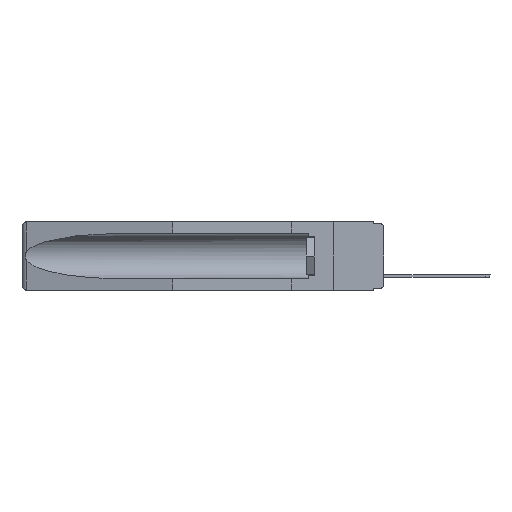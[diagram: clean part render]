
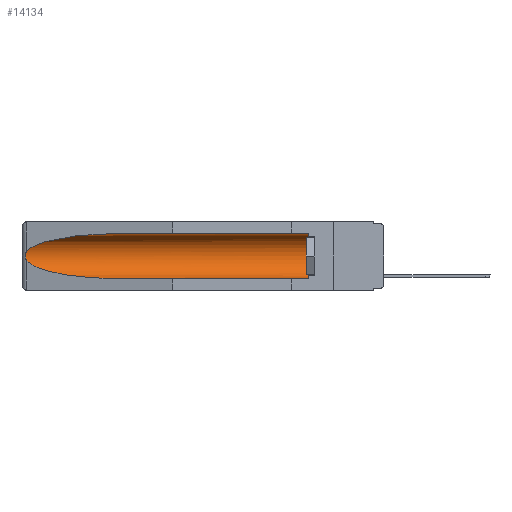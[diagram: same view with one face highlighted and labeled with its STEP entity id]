
A CAD part, left-side view. The second image highlights one B-rep face of the part: STEP entity #14134.
In plain terms, the highlighted cylindrical face has radius 2.857 mm (diameter 5.715 mm), a partial arc.
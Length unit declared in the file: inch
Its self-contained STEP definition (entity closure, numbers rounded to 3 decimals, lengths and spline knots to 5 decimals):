
#283 = EDGE_CURVE ( 'NONE', #15551, #11050, #1212, .T. ) ;
#292 = CARTESIAN_POINT ( 'NONE',  ( 0.26597, 1.5296, -0.19026 ) ) ;
#333 = CARTESIAN_POINT ( 'NONE',  ( 0.155, 1.07973, -0.284 ) ) ;
#392 = CARTESIAN_POINT ( 'NONE',  ( 0.155, 0.126, -0.1715 ) ) ;
#1212 =( BOUNDED_CURVE ( )  B_SPLINE_CURVE ( 3, ( #18219, #14955, #18429, #333 ),
 .UNSPECIFIED., .F., .F. ) 
 B_SPLINE_CURVE_WITH_KNOTS ( ( 4, 4 ),
 ( 0.1948, 1.5708 ),
 .UNSPECIFIED. ) 
 CURVE ( )  GEOMETRIC_REPRESENTATION_ITEM ( )  RATIONAL_B_SPLINE_CURVE ( ( 1., 0.848, 0.848, 1. ) ) 
 REPRESENTATION_ITEM ( '' )  );
#1786 = DIRECTION ( 'NONE',  ( 0., 0., 1. ) ) ;
#2035 = DIRECTION ( 'NONE',  ( 0., 0., 1. ) ) ;
#4675 = DIRECTION ( 'NONE',  ( 0., 1., 0. ) ) ;
#5060 = FACE_OUTER_BOUND ( 'NONE', #14733, .T. ) ;
#5086 = CARTESIAN_POINT ( 'NONE',  ( 0.26537, 1.52718, -0.19328 ) ) ;
#5282 = CARTESIAN_POINT ( 'NONE',  ( 0.26654, 1.53092, -0.15636 ) ) ;
#5899 = EDGE_CURVE ( 'NONE', #21203, #11050, #11670, .T. ) ;
#6003 = CARTESIAN_POINT ( 'NONE',  ( 0.26537, 1.52718, -0.14972 ) ) ;
#6364 = CARTESIAN_POINT ( 'NONE',  ( 0.26537, 1.52718, -0.19328 ) ) ;
#7251 = AXIS2_PLACEMENT_3D ( 'NONE', #392, #8354, #2035 ) ;
#7494 = VERTEX_POINT ( 'NONE', #12966 ) ;
#7540 = CARTESIAN_POINT ( 'NONE',  ( 0.21114, 1.30732, -0.059 ) ) ;
#7868 = ORIENTED_EDGE ( 'NONE', *, *, #19672, .T. ) ;
#7969 = ORIENTED_EDGE ( 'NONE', *, *, #15896, .T. ) ;
#8354 = DIRECTION ( 'NONE',  ( 0., -1., 0. ) ) ;
#8452 = CARTESIAN_POINT ( 'NONE',  ( 0.26597, 1.52961, -0.15275 ) ) ;
#8884 = CARTESIAN_POINT ( 'NONE',  ( 0.2673, 1.5327, -0.16383 ) ) ;
#8929 = ORIENTED_EDGE ( 'NONE', *, *, #16519, .T. ) ;
#9160 = CARTESIAN_POINT ( 'NONE',  ( 0.155, 1.07973, -0.059 ) ) ;
#10077 = ORIENTED_EDGE ( 'NONE', *, *, #12152, .T. ) ;
#10085 = CARTESIAN_POINT ( 'NONE',  ( 0.26655, 1.53094, -0.18657 ) ) ;
#11050 = VERTEX_POINT ( 'NONE', #17052 ) ;
#11521 = LINE ( 'NONE', #21470, #18979 ) ;
#11670 = LINE ( 'NONE', #13609, #13243 ) ;
#11712 = CARTESIAN_POINT ( 'NONE',  ( 0.155, -0.30754, -0.1715 ) ) ;
#12152 = EDGE_CURVE ( 'NONE', #16739, #17936, #11521, .T. ) ;
#12517 = ORIENTED_EDGE ( 'NONE', *, *, #5899, .F. ) ;
#12966 = CARTESIAN_POINT ( 'NONE',  ( 0.26537, 1.52718, -0.14972 ) ) ;
#13243 = VECTOR ( 'NONE', #18323, 39.37008 ) ;
#13474 = CARTESIAN_POINT ( 'NONE',  ( 0.26537, 1.52718, -0.14972 ) ) ;
#13591 = CARTESIAN_POINT ( 'NONE',  ( 0.155, 1.07973, -0.059 ) ) ;
#13609 = CARTESIAN_POINT ( 'NONE',  ( 0.155, -0.30754, -0.284 ) ) ;
#14134 = ADVANCED_FACE ( 'NONE', ( #5060 ), #20427, .F. ) ;
#14185 = CARTESIAN_POINT ( 'NONE',  ( 0.25451, 1.48313, -0.09465 ) ) ;
#14733 = EDGE_LOOP ( 'NONE', ( #7969, #7868, #14762, #12517, #8929, #10077 ) ) ;
#14762 = ORIENTED_EDGE ( 'NONE', *, *, #283, .T. ) ;
#14955 = CARTESIAN_POINT ( 'NONE',  ( 0.25451, 1.48313, -0.24835 ) ) ;
#15151 = B_SPLINE_CURVE_WITH_KNOTS ( 'NONE', 3,
 ( #13474, #8452, #5282, #8884, #20228, #16975, #20032, #10085, #292, #5086 ),
 .UNSPECIFIED., .F., .F.,
 ( 4, 2, 2, 2, 4 ),
 ( 0., 0.00029, 0.00058, 0.00087, 0.00117 ),
 .UNSPECIFIED. ) ;
#15551 = VERTEX_POINT ( 'NONE', #6364 ) ;
#15896 = EDGE_CURVE ( 'NONE', #17936, #7494, #20554, .T. ) ;
#16240 = AXIS2_PLACEMENT_3D ( 'NONE', #11712, #18362, #1786 ) ;
#16519 = EDGE_CURVE ( 'NONE', #21203, #16739, #16669, .T. ) ;
#16669 = CIRCLE ( 'NONE', #7251, 0.1125 ) ;
#16739 = VERTEX_POINT ( 'NONE', #18708 ) ;
#16975 = CARTESIAN_POINT ( 'NONE',  ( 0.2675, 1.53308, -0.17534 ) ) ;
#17052 = CARTESIAN_POINT ( 'NONE',  ( 0.155, 1.07973, -0.284 ) ) ;
#17936 = VERTEX_POINT ( 'NONE', #13591 ) ;
#18219 = CARTESIAN_POINT ( 'NONE',  ( 0.26537, 1.52718, -0.19328 ) ) ;
#18323 = DIRECTION ( 'NONE',  ( 0., 1., 0. ) ) ;
#18362 = DIRECTION ( 'NONE',  ( 0., 1., 0. ) ) ;
#18429 = CARTESIAN_POINT ( 'NONE',  ( 0.21114, 1.30732, -0.284 ) ) ;
#18708 = CARTESIAN_POINT ( 'NONE',  ( 0.155, 0.126, -0.059 ) ) ;
#18979 = VECTOR ( 'NONE', #4675, 39.37008 ) ;
#19382 = CARTESIAN_POINT ( 'NONE',  ( 0.155, 0.126, -0.284 ) ) ;
#19672 = EDGE_CURVE ( 'NONE', #7494, #15551, #15151, .T. ) ;
#20032 = CARTESIAN_POINT ( 'NONE',  ( 0.2673, 1.53269, -0.17917 ) ) ;
#20228 = CARTESIAN_POINT ( 'NONE',  ( 0.2675, 1.53308, -0.16763 ) ) ;
#20427 = CYLINDRICAL_SURFACE ( 'NONE', #16240, 0.1125 ) ;
#20554 =( BOUNDED_CURVE ( )  B_SPLINE_CURVE ( 3, ( #9160, #7540, #14185, #6003 ),
 .UNSPECIFIED., .F., .F. ) 
 B_SPLINE_CURVE_WITH_KNOTS ( ( 4, 4 ),
 ( 4.71239, 6.08839 ),
 .UNSPECIFIED. ) 
 CURVE ( )  GEOMETRIC_REPRESENTATION_ITEM ( )  RATIONAL_B_SPLINE_CURVE ( ( 1., 0.848, 0.848, 1. ) ) 
 REPRESENTATION_ITEM ( '' )  );
#21203 = VERTEX_POINT ( 'NONE', #19382 ) ;
#21470 = CARTESIAN_POINT ( 'NONE',  ( 0.155, -0.30754, -0.059 ) ) ;
